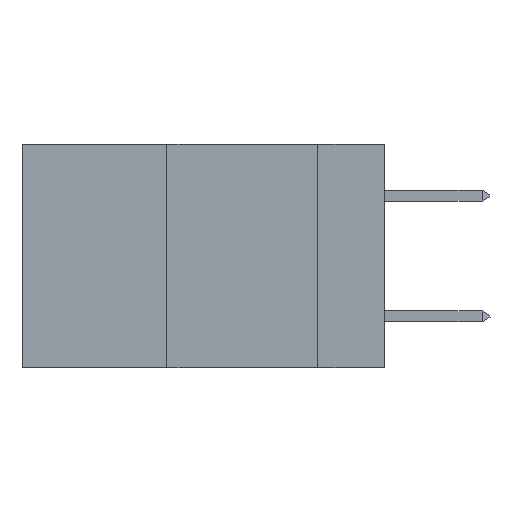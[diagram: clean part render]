
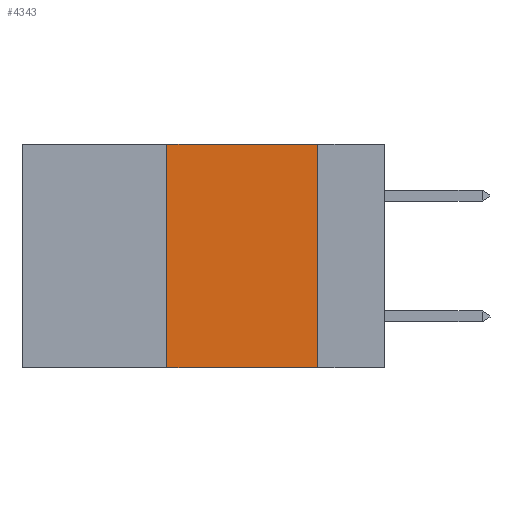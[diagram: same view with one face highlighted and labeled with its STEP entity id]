
A CAD part, left-side view. The second image highlights one B-rep face of the part: STEP entity #4343.
In plain terms, the highlighted planar face has unit normal (-1, 0, 0).
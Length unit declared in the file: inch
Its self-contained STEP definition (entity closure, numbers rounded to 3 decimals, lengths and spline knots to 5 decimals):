
#188 = FACE_OUTER_BOUND ( 'NONE', #18797, .T. ) ;
#638 = VECTOR ( 'NONE', #3165, 39.37008 ) ;
#1184 = LINE ( 'NONE', #19674, #19820 ) ;
#3165 = DIRECTION ( 'NONE',  ( 0., -1., 0. ) ) ;
#3369 = ORIENTED_EDGE ( 'NONE', *, *, #6642, .F. ) ;
#4206 = VERTEX_POINT ( 'NONE', #4626 ) ;
#4343 = ADVANCED_FACE ( 'NONE', ( #188 ), #17687, .F. ) ;
#4626 = CARTESIAN_POINT ( 'NONE',  ( 0., 0.36, -0.37 ) ) ;
#5179 = CARTESIAN_POINT ( 'NONE',  ( 0., 0.6, 0. ) ) ;
#5458 = LINE ( 'NONE', #6719, #638 ) ;
#5566 = LINE ( 'NONE', #5179, #9820 ) ;
#6130 = CARTESIAN_POINT ( 'NONE',  ( 0., 0.11, -0.37 ) ) ;
#6642 = EDGE_CURVE ( 'NONE', #14407, #16788, #9480, .T. ) ;
#6719 = CARTESIAN_POINT ( 'NONE',  ( 0., 0.6, -0.37 ) ) ;
#7668 = DIRECTION ( 'NONE',  ( 0., 0., -1. ) ) ;
#7914 = CARTESIAN_POINT ( 'NONE',  ( 0., 0.36, 0. ) ) ;
#8220 = ORIENTED_EDGE ( 'NONE', *, *, #11946, .F. ) ;
#8659 = DIRECTION ( 'NONE',  ( 1., 0., 0. ) ) ;
#9480 = LINE ( 'NONE', #18572, #17962 ) ;
#9820 = VECTOR ( 'NONE', #21347, 39.37008 ) ;
#10697 = DIRECTION ( 'NONE',  ( 0., 0., 1. ) ) ;
#11946 = EDGE_CURVE ( 'NONE', #4206, #12561, #1184, .T. ) ;
#12561 = VERTEX_POINT ( 'NONE', #7914 ) ;
#14407 = VERTEX_POINT ( 'NONE', #16530 ) ;
#14909 = EDGE_CURVE ( 'NONE', #12561, #14407, #5566, .T. ) ;
#15321 = ORIENTED_EDGE ( 'NONE', *, *, #14909, .F. ) ;
#16419 = AXIS2_PLACEMENT_3D ( 'NONE', #19452, #8659, #21265 ) ;
#16530 = CARTESIAN_POINT ( 'NONE',  ( 0., 0.11, 0. ) ) ;
#16788 = VERTEX_POINT ( 'NONE', #6130 ) ;
#17687 = PLANE ( 'NONE',  #16419 ) ;
#17962 = VECTOR ( 'NONE', #7668, 39.37008 ) ;
#18572 = CARTESIAN_POINT ( 'NONE',  ( 0., 0.11, 0. ) ) ;
#18797 = EDGE_LOOP ( 'NONE', ( #3369, #15321, #8220, #21516 ) ) ;
#19452 = CARTESIAN_POINT ( 'NONE',  ( 0., 0.6, 0. ) ) ;
#19674 = CARTESIAN_POINT ( 'NONE',  ( 0., 0.36, 0. ) ) ;
#19820 = VECTOR ( 'NONE', #10697, 39.37008 ) ;
#21265 = DIRECTION ( 'NONE',  ( 0., 0., -1. ) ) ;
#21286 = EDGE_CURVE ( 'NONE', #4206, #16788, #5458, .T. ) ;
#21347 = DIRECTION ( 'NONE',  ( 0., -1., 0. ) ) ;
#21516 = ORIENTED_EDGE ( 'NONE', *, *, #21286, .T. ) ;
